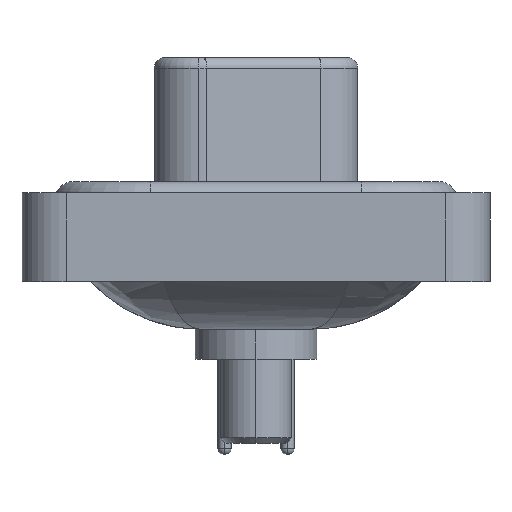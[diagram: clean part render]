
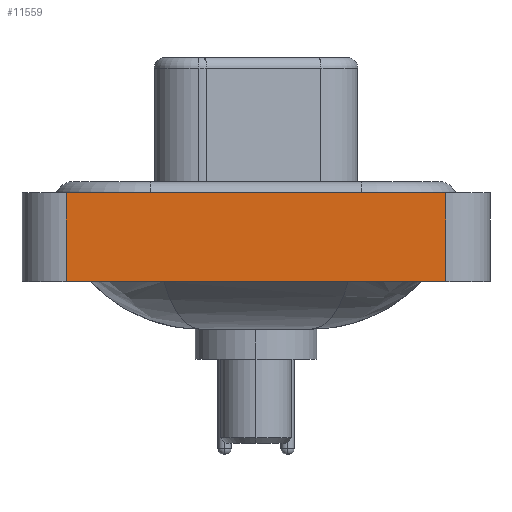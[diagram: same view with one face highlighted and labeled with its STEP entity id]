
A CAD part, left-side view. The second image highlights one B-rep face of the part: STEP entity #11559.
In plain terms, the highlighted planar face has unit normal (-1, 0, 0).
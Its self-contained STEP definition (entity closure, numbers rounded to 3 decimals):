
#27 = DIRECTION ( 'NONE',  ( 0., 0., 1. ) ) ;
#96 = CARTESIAN_POINT ( 'NONE',  ( -7.35, -8.55, 0.4 ) ) ;
#482 = CARTESIAN_POINT ( 'NONE',  ( -7.35, -8.55, -3.6 ) ) ;
#603 = LINE ( 'NONE', #6965, #6444 ) ;
#1907 = CARTESIAN_POINT ( 'NONE',  ( -7.35, -8.55, -3.6 ) ) ;
#2217 = VERTEX_POINT ( 'NONE', #4524 ) ;
#3818 = VERTEX_POINT ( 'NONE', #19783 ) ;
#4265 = VECTOR ( 'NONE', #8519, 1000. ) ;
#4524 = CARTESIAN_POINT ( 'NONE',  ( -7.35, 8.55, -3.6 ) ) ;
#5183 = ORIENTED_EDGE ( 'NONE', *, *, #19231, .T. ) ;
#6228 = EDGE_CURVE ( 'NONE', #2217, #3818, #603, .T. ) ;
#6444 = VECTOR ( 'NONE', #13352, 1000. ) ;
#6965 = CARTESIAN_POINT ( 'NONE',  ( -7.35, 8.55, -3.6 ) ) ;
#8282 = DIRECTION ( 'NONE',  ( 0., 0., 1. ) ) ;
#8319 = ORIENTED_EDGE ( 'NONE', *, *, #16207, .F. ) ;
#8519 = DIRECTION ( 'NONE',  ( 0., -1., 0. ) ) ;
#9210 = FACE_OUTER_BOUND ( 'NONE', #19573, .T. ) ;
#9526 = LINE ( 'NONE', #14335, #9997 ) ;
#9629 = CARTESIAN_POINT ( 'NONE',  ( -7.35, -8.55, -3.6 ) ) ;
#9997 = VECTOR ( 'NONE', #11107, 1000. ) ;
#10189 = LINE ( 'NONE', #16575, #4265 ) ;
#11107 = DIRECTION ( 'NONE',  ( 0., -1., 0. ) ) ;
#11315 = EDGE_CURVE ( 'NONE', #2217, #20249, #10189, .T. ) ;
#11333 = AXIS2_PLACEMENT_3D ( 'NONE', #9629, #16031, #27 ) ;
#11559 = ADVANCED_FACE ( 'NONE', ( #9210 ), #20618, .T. ) ;
#12337 = ORIENTED_EDGE ( 'NONE', *, *, #11315, .T. ) ;
#12455 = ORIENTED_EDGE ( 'NONE', *, *, #6228, .F. ) ;
#13352 = DIRECTION ( 'NONE',  ( 0., 0., 1. ) ) ;
#14335 = CARTESIAN_POINT ( 'NONE',  ( -7.35, -8.55, 0.4 ) ) ;
#16031 = DIRECTION ( 'NONE',  ( -1., 0., 0. ) ) ;
#16207 = EDGE_CURVE ( 'NONE', #3818, #18143, #9526, .T. ) ;
#16496 = VECTOR ( 'NONE', #8282, 1000. ) ;
#16575 = CARTESIAN_POINT ( 'NONE',  ( -7.35, -8.55, -3.6 ) ) ;
#17701 = LINE ( 'NONE', #1907, #16496 ) ;
#18143 = VERTEX_POINT ( 'NONE', #96 ) ;
#19231 = EDGE_CURVE ( 'NONE', #20249, #18143, #17701, .T. ) ;
#19573 = EDGE_LOOP ( 'NONE', ( #5183, #8319, #12455, #12337 ) ) ;
#19783 = CARTESIAN_POINT ( 'NONE',  ( -7.35, 8.55, 0.4 ) ) ;
#20249 = VERTEX_POINT ( 'NONE', #482 ) ;
#20618 = PLANE ( 'NONE',  #11333 ) ;
